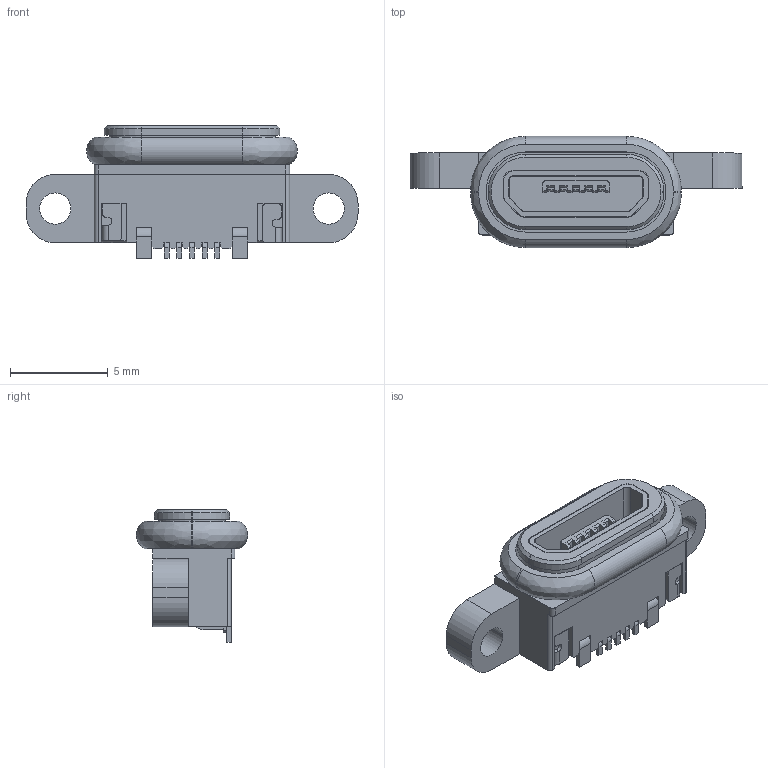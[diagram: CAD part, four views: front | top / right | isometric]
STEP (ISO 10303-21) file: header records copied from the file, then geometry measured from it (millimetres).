
FILE_DESCRIPTION (( 'STEP AP214' ), '1' );
FILE_NAME ('690-W05-290-483.STEP', '2021-04-13T15:28:36', ( '' ), ( '' ), 'SwSTEP 2.0', 'SolidWorks 2020', '' );
FILE_SCHEMA (( 'AUTOMOTIVE_DESIGN' ));
Length unit declared in the file: millimetre
Products named in the file (6): HOUSING 690-W05-X90-483; CONTACTS 690-W05-X90-483; SHELL 690-W05-X90-483; O-RING 690-W05-X90-483; SOLDER PADS 690-W05-X90-483; 690-W05-290-483
Assembly tree (5 placements, depth 2):
  690-W05-290-483
    HOUSING 690-W05-X90-483
    CONTACTS 690-W05-X90-483
    SHELL 690-W05-X90-483
    SOLDER PADS 690-W05-X90-483
    O-RING 690-W05-X90-483
Bounding box: 17 x 5.69 x 6.8 mm (x, y, z)
Volume: 214 mm3; surface area: 827.6 mm2
Topology: 10 solids, 10 shells, 637 faces, 1804 edges, 1183 vertices
Faces by surface type: plane 452, cylinder 177, cone 4, bspline 4
Entity records: 20903 total; most frequent: CARTESIAN_POINT 3722, ORIENTED_EDGE 3608, DIRECTION 3434, EDGE_CURVE 1804, VECTOR 1436, LINE 1436, VERTEX_POINT 1183, AXIS2_PLACEMENT_3D 999
